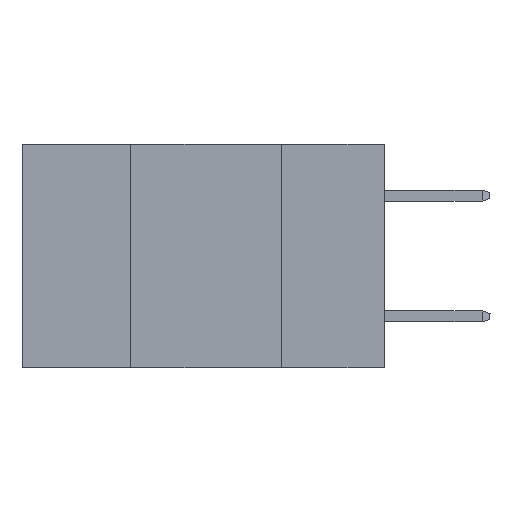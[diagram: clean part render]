
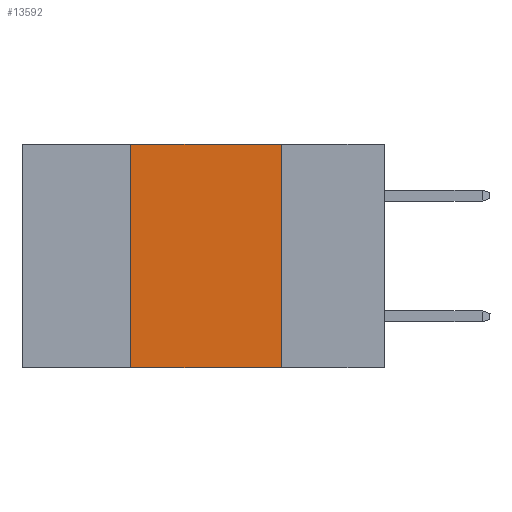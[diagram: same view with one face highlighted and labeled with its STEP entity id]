
A CAD part, left-side view. The second image highlights one B-rep face of the part: STEP entity #13592.
In plain terms, the highlighted planar face has unit normal (-1, 0, 0).
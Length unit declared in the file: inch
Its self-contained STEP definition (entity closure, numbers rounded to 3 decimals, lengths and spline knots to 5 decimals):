
#9 = CARTESIAN_POINT ( 'NONE',  ( 0., 0.42, 0. ) ) ;
#280 = ORIENTED_EDGE ( 'NONE', *, *, #14036, .T. ) ;
#1423 = CARTESIAN_POINT ( 'NONE',  ( 0., 0.17, 0. ) ) ;
#1558 = DIRECTION ( 'NONE',  ( 0., -1., 0. ) ) ;
#2146 = CARTESIAN_POINT ( 'NONE',  ( 0., 0.6, -0.37 ) ) ;
#2307 = DIRECTION ( 'NONE',  ( 0., -1., 0. ) ) ;
#2543 = EDGE_LOOP ( 'NONE', ( #11225, #5954, #13743, #280 ) ) ;
#3359 = EDGE_CURVE ( 'NONE', #4838, #15956, #4103, .T. ) ;
#3633 = LINE ( 'NONE', #2146, #5812 ) ;
#4103 = LINE ( 'NONE', #7718, #5703 ) ;
#4286 = EDGE_CURVE ( 'NONE', #15956, #5490, #10109, .T. ) ;
#4838 = VERTEX_POINT ( 'NONE', #11748 ) ;
#5490 = VERTEX_POINT ( 'NONE', #14527 ) ;
#5703 = VECTOR ( 'NONE', #1558, 39.37008 ) ;
#5812 = VECTOR ( 'NONE', #2307, 39.37008 ) ;
#5954 = ORIENTED_EDGE ( 'NONE', *, *, #3359, .F. ) ;
#7718 = CARTESIAN_POINT ( 'NONE',  ( 0., 0.6, 0. ) ) ;
#7742 = PLANE ( 'NONE',  #13462 ) ;
#7916 = DIRECTION ( 'NONE',  ( 0., 0., -1. ) ) ;
#10109 = LINE ( 'NONE', #1423, #12512 ) ;
#10137 = DIRECTION ( 'NONE',  ( 0., 0., -1. ) ) ;
#10340 = DIRECTION ( 'NONE',  ( 0., 0., 1. ) ) ;
#11225 = ORIENTED_EDGE ( 'NONE', *, *, #4286, .F. ) ;
#11286 = VERTEX_POINT ( 'NONE', #13095 ) ;
#11748 = CARTESIAN_POINT ( 'NONE',  ( 0., 0.42, 0. ) ) ;
#12512 = VECTOR ( 'NONE', #7916, 39.37008 ) ;
#12879 = CARTESIAN_POINT ( 'NONE',  ( 0., 0.6, 0. ) ) ;
#13016 = FACE_OUTER_BOUND ( 'NONE', #2543, .T. ) ;
#13032 = VECTOR ( 'NONE', #10340, 39.37008 ) ;
#13095 = CARTESIAN_POINT ( 'NONE',  ( 0., 0.42, -0.37 ) ) ;
#13165 = EDGE_CURVE ( 'NONE', #11286, #4838, #16459, .T. ) ;
#13462 = AXIS2_PLACEMENT_3D ( 'NONE', #12879, #14068, #10137 ) ;
#13592 = ADVANCED_FACE ( 'NONE', ( #13016 ), #7742, .F. ) ;
#13743 = ORIENTED_EDGE ( 'NONE', *, *, #13165, .F. ) ;
#14036 = EDGE_CURVE ( 'NONE', #11286, #5490, #3633, .T. ) ;
#14068 = DIRECTION ( 'NONE',  ( 1., 0., 0. ) ) ;
#14527 = CARTESIAN_POINT ( 'NONE',  ( 0., 0.17, -0.37 ) ) ;
#15844 = CARTESIAN_POINT ( 'NONE',  ( 0., 0.17, 0. ) ) ;
#15956 = VERTEX_POINT ( 'NONE', #15844 ) ;
#16459 = LINE ( 'NONE', #9, #13032 ) ;
